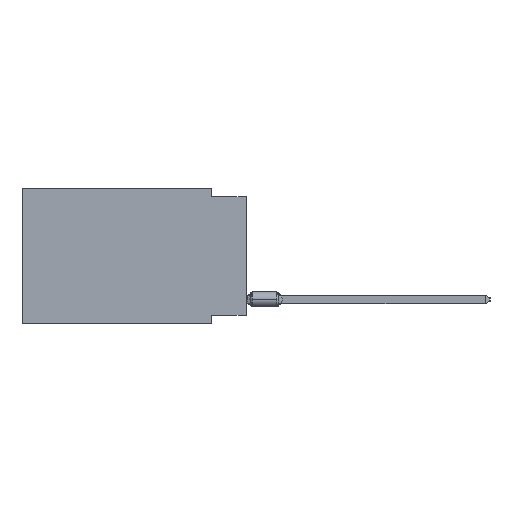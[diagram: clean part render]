
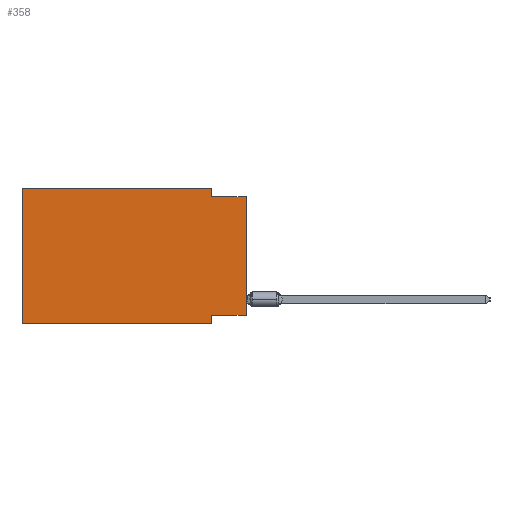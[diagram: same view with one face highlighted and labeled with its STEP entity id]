
A CAD part, left-side view. The second image highlights one B-rep face of the part: STEP entity #358.
In plain terms, the highlighted planar face has unit normal (-1, 0, 0).
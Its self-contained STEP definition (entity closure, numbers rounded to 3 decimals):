
#358 = ADVANCED_FACE ( 'NONE', ( #10209 ), #6094, .F. ) ;
#797 = LINE ( 'NONE', #34198, #7572 ) ;
#825 = LINE ( 'NONE', #30125, #42215 ) ;
#1234 = VERTEX_POINT ( 'NONE', #16811 ) ;
#1370 = CARTESIAN_POINT ( 'NONE',  ( 0., 0., -9.271 ) ) ;
#2245 = VERTEX_POINT ( 'NONE', #33431 ) ;
#2706 = EDGE_LOOP ( 'NONE', ( #26912, #42126, #27202, #29663, #37929, #29785, #35010, #19038 ) ) ;
#3093 = EDGE_CURVE ( 'NONE', #4822, #1234, #29783, .T. ) ;
#3484 = DIRECTION ( 'NONE',  ( 0., 0., -1. ) ) ;
#3967 = AXIS2_PLACEMENT_3D ( 'NONE', #16486, #16072, #3484 ) ;
#4345 = CARTESIAN_POINT ( 'NONE',  ( 0., 0., -0.635 ) ) ;
#4822 = VERTEX_POINT ( 'NONE', #32442 ) ;
#5164 = LINE ( 'NONE', #11687, #12509 ) ;
#6094 = PLANE ( 'NONE',  #3967 ) ;
#6249 = EDGE_CURVE ( 'NONE', #32310, #34066, #797, .T. ) ;
#7572 = VECTOR ( 'NONE', #27260, 1000. ) ;
#10175 = CARTESIAN_POINT ( 'NONE',  ( 0., 0., -0.635 ) ) ;
#10209 = FACE_OUTER_BOUND ( 'NONE', #2706, .T. ) ;
#10947 = EDGE_CURVE ( 'NONE', #1234, #16150, #19493, .T. ) ;
#11000 = EDGE_CURVE ( 'NONE', #38618, #16150, #37280, .T. ) ;
#11687 = CARTESIAN_POINT ( 'NONE',  ( 0., 16.383, 0. ) ) ;
#12472 = VECTOR ( 'NONE', #39315, 1000. ) ;
#12509 = VECTOR ( 'NONE', #30765, 1000. ) ;
#13622 = EDGE_CURVE ( 'NONE', #25297, #2245, #825, .T. ) ;
#13804 = VECTOR ( 'NONE', #40119, 1000. ) ;
#14262 = CARTESIAN_POINT ( 'NONE',  ( 0., 0., 0. ) ) ;
#14289 = EDGE_CURVE ( 'NONE', #38618, #25297, #27981, .T. ) ;
#14531 = DIRECTION ( 'NONE',  ( 0., 1., 0. ) ) ;
#16072 = DIRECTION ( 'NONE',  ( 1., 0., 0. ) ) ;
#16150 = VERTEX_POINT ( 'NONE', #4345 ) ;
#16486 = CARTESIAN_POINT ( 'NONE',  ( 0., 16.383, 0. ) ) ;
#16811 = CARTESIAN_POINT ( 'NONE',  ( 0., 2.54, -0.635 ) ) ;
#18016 = VECTOR ( 'NONE', #14531, 1000. ) ;
#18118 = CARTESIAN_POINT ( 'NONE',  ( 0., 16.383, -9.906 ) ) ;
#19038 = ORIENTED_EDGE ( 'NONE', *, *, #14289, .F. ) ;
#19343 = CARTESIAN_POINT ( 'NONE',  ( 0., 16.383, -9.906 ) ) ;
#19493 = LINE ( 'NONE', #10175, #13804 ) ;
#20680 = EDGE_CURVE ( 'NONE', #32310, #2245, #30192, .T. ) ;
#24726 = CARTESIAN_POINT ( 'NONE',  ( 0., 0., -9.271 ) ) ;
#25297 = VERTEX_POINT ( 'NONE', #32488 ) ;
#26912 = ORIENTED_EDGE ( 'NONE', *, *, #11000, .T. ) ;
#27092 = DIRECTION ( 'NONE',  ( 0., 0., -1. ) ) ;
#27202 = ORIENTED_EDGE ( 'NONE', *, *, #3093, .F. ) ;
#27260 = DIRECTION ( 'NONE',  ( 0., 0., 1. ) ) ;
#27981 = LINE ( 'NONE', #24726, #18016 ) ;
#29663 = ORIENTED_EDGE ( 'NONE', *, *, #40605, .F. ) ;
#29783 = LINE ( 'NONE', #36072, #12472 ) ;
#29785 = ORIENTED_EDGE ( 'NONE', *, *, #20680, .T. ) ;
#30125 = CARTESIAN_POINT ( 'NONE',  ( 0., 2.54, -9.906 ) ) ;
#30192 = LINE ( 'NONE', #19343, #30877 ) ;
#30765 = DIRECTION ( 'NONE',  ( 0., -1., 0. ) ) ;
#30877 = VECTOR ( 'NONE', #40185, 1000. ) ;
#32310 = VERTEX_POINT ( 'NONE', #18118 ) ;
#32442 = CARTESIAN_POINT ( 'NONE',  ( 0., 2.54, 0. ) ) ;
#32488 = CARTESIAN_POINT ( 'NONE',  ( 0., 2.54, -9.271 ) ) ;
#33431 = CARTESIAN_POINT ( 'NONE',  ( 0., 2.54, -9.906 ) ) ;
#34066 = VERTEX_POINT ( 'NONE', #38317 ) ;
#34198 = CARTESIAN_POINT ( 'NONE',  ( 0., 16.383, 0. ) ) ;
#34454 = DIRECTION ( 'NONE',  ( 0., 0., 1. ) ) ;
#35010 = ORIENTED_EDGE ( 'NONE', *, *, #13622, .F. ) ;
#36072 = CARTESIAN_POINT ( 'NONE',  ( 0., 2.54, 0. ) ) ;
#36108 = VECTOR ( 'NONE', #34454, 1000. ) ;
#37280 = LINE ( 'NONE', #14262, #36108 ) ;
#37929 = ORIENTED_EDGE ( 'NONE', *, *, #6249, .F. ) ;
#38317 = CARTESIAN_POINT ( 'NONE',  ( 0., 16.383, 0. ) ) ;
#38618 = VERTEX_POINT ( 'NONE', #1370 ) ;
#39315 = DIRECTION ( 'NONE',  ( 0., 0., -1. ) ) ;
#40119 = DIRECTION ( 'NONE',  ( 0., -1., 0. ) ) ;
#40185 = DIRECTION ( 'NONE',  ( 0., -1., 0. ) ) ;
#40605 = EDGE_CURVE ( 'NONE', #34066, #4822, #5164, .T. ) ;
#42126 = ORIENTED_EDGE ( 'NONE', *, *, #10947, .F. ) ;
#42215 = VECTOR ( 'NONE', #27092, 1000. ) ;
